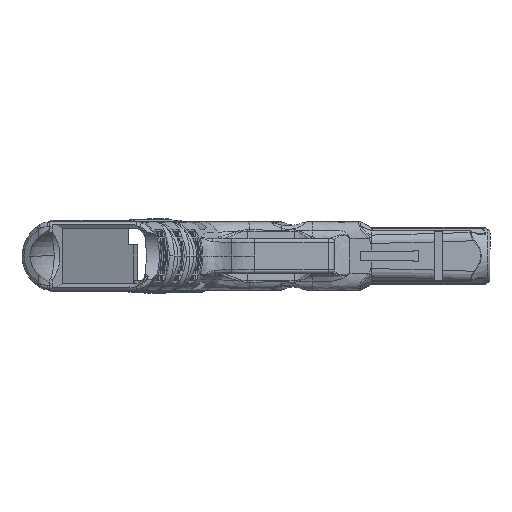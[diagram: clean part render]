
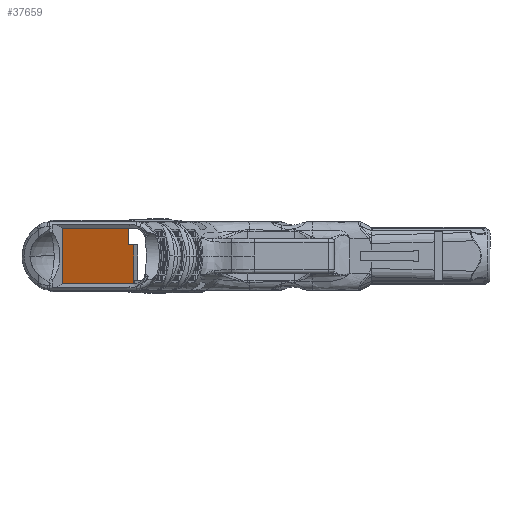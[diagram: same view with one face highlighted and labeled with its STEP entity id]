
A CAD part, front view. The second image highlights one B-rep face of the part: STEP entity #37659.
In plain terms, the highlighted planar face has unit normal (0.95, -0.311, 0).
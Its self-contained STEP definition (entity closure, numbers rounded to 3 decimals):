
#195=PLANE('',#40023);
#2650=FACE_OUTER_BOUND('',#4794,.T.);
#4794=EDGE_LOOP('',(#27228,#27229,#27230,#27231,#27232,#27233,#27234,#27235));
#7067=LINE('',#53873,#9589);
#7072=LINE('',#53881,#9594);
#7073=LINE('',#53884,#9595);
#7077=LINE('',#53891,#9599);
#7228=LINE('',#54447,#9750);
#7346=LINE('',#56974,#9868);
#7455=LINE('',#74227,#9977);
#7739=LINE('',#88729,#10261);
#9589=VECTOR('',#41960,1.);
#9594=VECTOR('',#41967,10.);
#9595=VECTOR('',#41970,1.);
#9599=VECTOR('',#41976,1.);
#9750=VECTOR('',#42245,1.);
#9868=VECTOR('',#42571,1.);
#9977=VECTOR('',#42900,1.);
#10261=VECTOR('',#43686,1.);
#14841=VERTEX_POINT('',#53870);
#14842=VERTEX_POINT('',#53872);
#14844=VERTEX_POINT('',#53879);
#14845=VERTEX_POINT('',#53883);
#14847=VERTEX_POINT('',#53889);
#14849=VERTEX_POINT('',#53897);
#14999=VERTEX_POINT('',#54420);
#15004=VERTEX_POINT('',#54446);
#18813=EDGE_CURVE('',#14842,#14841,#7067,.T.);
#18818=EDGE_CURVE('',#14844,#14841,#7072,.T.);
#18819=EDGE_CURVE('',#14844,#14845,#7073,.T.);
#18823=EDGE_CURVE('',#14845,#14847,#7077,.T.);
#19010=EDGE_CURVE('',#15004,#14847,#7228,.T.);
#19217=EDGE_CURVE('',#14999,#15004,#7346,.T.);
#19576=EDGE_CURVE('',#14999,#14849,#7455,.T.);
#20271=EDGE_CURVE('',#14849,#14842,#7739,.T.);
#27228=ORIENTED_EDGE('',*,*,#18823,.T.);
#27229=ORIENTED_EDGE('',*,*,#19010,.F.);
#27230=ORIENTED_EDGE('',*,*,#19217,.F.);
#27231=ORIENTED_EDGE('',*,*,#19576,.T.);
#27232=ORIENTED_EDGE('',*,*,#20271,.T.);
#27233=ORIENTED_EDGE('',*,*,#18813,.T.);
#27234=ORIENTED_EDGE('',*,*,#18818,.F.);
#27235=ORIENTED_EDGE('',*,*,#18819,.T.);
#37659=ADVANCED_FACE('',(#2650),#195,.T.);
#40023=AXIS2_PLACEMENT_3D('',#88728,#43684,#43685);
#41960=DIRECTION('',(0.,0.,1.));
#41967=DIRECTION('',(0.311,0.95,0.));
#41970=DIRECTION('',(0.,0.,1.));
#41976=DIRECTION('',(-0.311,-0.95,0.));
#42245=DIRECTION('',(0.,0.,-1.));
#42571=DIRECTION('',(0.311,0.95,0.));
#42900=DIRECTION('',(0.,0.,-1.));
#43684=DIRECTION('center_axis',(0.95,-0.311,0.));
#43685=DIRECTION('ref_axis',(0.,0.,
1.));
#43686=DIRECTION('',(0.311,0.95,0.));
#53870=CARTESIAN_POINT('',(32.453,-5.967,-10.375));
#53872=CARTESIAN_POINT('',(32.453,-5.967,-11.75));
#53873=CARTESIAN_POINT('',(32.453,-5.967,-11.75));
#53879=CARTESIAN_POINT('',(32.448,-5.982,-10.375));
#53881=CARTESIAN_POINT('',(32.119,-6.987,-10.375));
#53883=CARTESIAN_POINT('',(32.448,-5.982,4.75));
#53884=CARTESIAN_POINT('',(32.448,-5.982,-11.75));
#53889=CARTESIAN_POINT('',(30.347,-12.4,4.75));
#53891=CARTESIAN_POINT('',(18.858,-47.499,4.75));
#53897=CARTESIAN_POINT('',(2.327,-98.,-11.75));
#54420=CARTESIAN_POINT('',(2.327,-98.,11.75));
#54446=CARTESIAN_POINT('',(30.347,-12.4,11.75));
#54447=CARTESIAN_POINT('',(30.347,-12.4,2.982));
#56974=CARTESIAN_POINT('',(2.,-99.,11.75));
#74227=CARTESIAN_POINT('',(2.327,-98.,-18.375));
#88728=CARTESIAN_POINT('Origin',(2.,-99.,-11.75));
#88729=CARTESIAN_POINT('',(2.,-99.,-11.75));
